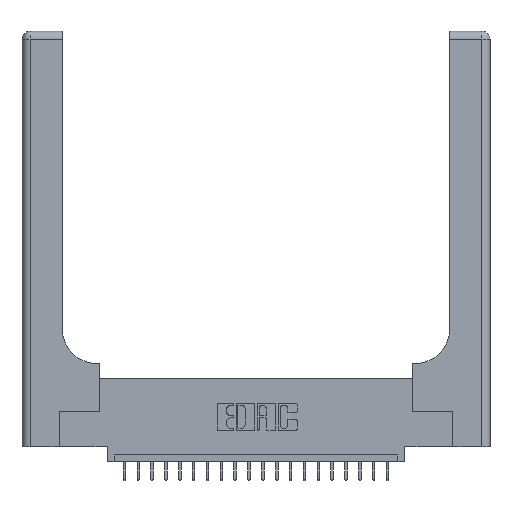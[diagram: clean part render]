
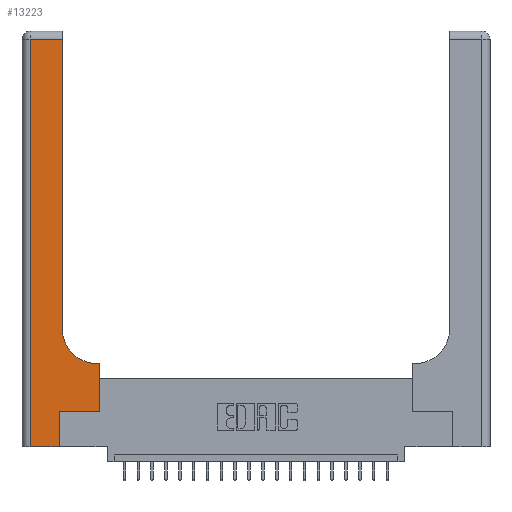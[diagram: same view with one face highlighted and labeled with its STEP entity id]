
A CAD part, top view. The second image highlights one B-rep face of the part: STEP entity #13223.
In plain terms, the highlighted planar face has unit normal (0, 0, 1).
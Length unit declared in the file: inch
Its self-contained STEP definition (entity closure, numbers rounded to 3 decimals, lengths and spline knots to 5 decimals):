
#130 = ORIENTED_EDGE ( 'NONE', *, *, #7487, .T. ) ;
#332 = CARTESIAN_POINT ( 'NONE',  ( 0.06, 0., 0.37 ) ) ;
#352 = AXIS2_PLACEMENT_3D ( 'NONE', #9188, #16458, #19156 ) ;
#564 = EDGE_CURVE ( 'NONE', #5405, #22552, #14140, .T. ) ;
#884 = CARTESIAN_POINT ( 'NONE',  ( 0.5585, 0.6, 0.37 ) ) ;
#927 = DIRECTION ( 'NONE',  ( -1., 0., 0. ) ) ;
#1056 = CARTESIAN_POINT ( 'NONE',  ( 0.2915, 0.6, 0.37 ) ) ;
#1364 = CARTESIAN_POINT ( 'NONE',  ( 0.5585, 0.25, 0.37 ) ) ;
#1836 = PLANE ( 'NONE',  #352 ) ;
#2170 = VERTEX_POINT ( 'NONE', #17887 ) ;
#2450 = LINE ( 'NONE', #22140, #11781 ) ;
#2534 = EDGE_CURVE ( 'NONE', #4818, #21847, #2450, .T. ) ;
#3393 = VERTEX_POINT ( 'NONE', #13955 ) ;
#4415 = LINE ( 'NONE', #22246, #14226 ) ;
#4580 = VERTEX_POINT ( 'NONE', #332 ) ;
#4818 = VERTEX_POINT ( 'NONE', #6600 ) ;
#5195 = VECTOR ( 'NONE', #21370, 39.37008 ) ;
#5405 = VERTEX_POINT ( 'NONE', #1364 ) ;
#5787 = ORIENTED_EDGE ( 'NONE', *, *, #16520, .T. ) ;
#5951 = FACE_OUTER_BOUND ( 'NONE', #8430, .T. ) ;
#6069 = EDGE_CURVE ( 'NONE', #15256, #13187, #13491, .T. ) ;
#6600 = CARTESIAN_POINT ( 'NONE',  ( 0.269, 0., 0.37 ) ) ;
#7013 = DIRECTION ( 'NONE',  ( 0., 1., 0. ) ) ;
#7487 = EDGE_CURVE ( 'NONE', #21847, #5405, #16011, .T. ) ;
#7909 = CARTESIAN_POINT ( 'NONE',  ( 0., 2.94, 0.37 ) ) ;
#8078 = VECTOR ( 'NONE', #12597, 39.37008 ) ;
#8288 = VECTOR ( 'NONE', #21776, 39.37008 ) ;
#8430 = EDGE_LOOP ( 'NONE', ( #8604, #16390, #15786, #5787, #19103, #130, #19903, #15740, #17509 ) ) ;
#8604 = ORIENTED_EDGE ( 'NONE', *, *, #13156, .T. ) ;
#8641 = EDGE_CURVE ( 'NONE', #22552, #2170, #11867, .T. ) ;
#9188 = CARTESIAN_POINT ( 'NONE',  ( 0., 3., 0.37 ) ) ;
#9488 = EDGE_CURVE ( 'NONE', #13187, #4580, #4415, .T. ) ;
#10197 = DIRECTION ( 'NONE',  ( -1., 0., 0. ) ) ;
#10296 = CARTESIAN_POINT ( 'NONE',  ( 0.2915, 2.94, 0.37 ) ) ;
#10298 = VECTOR ( 'NONE', #927, 39.37008 ) ;
#10690 = CARTESIAN_POINT ( 'NONE',  ( 0.5585, 0.25, 0.37 ) ) ;
#11186 = DIRECTION ( 'NONE',  ( 0., 0., -1. ) ) ;
#11340 = CARTESIAN_POINT ( 'NONE',  ( 0.06, 2.94, 0.37 ) ) ;
#11781 = VECTOR ( 'NONE', #7013, 39.37008 ) ;
#11867 = LINE ( 'NONE', #1056, #14597 ) ;
#12467 = CARTESIAN_POINT ( 'NONE',  ( 0., 0., 0.37 ) ) ;
#12597 = DIRECTION ( 'NONE',  ( 1., 0., 0. ) ) ;
#12977 = CARTESIAN_POINT ( 'NONE',  ( 0.2915, 3., 0.37 ) ) ;
#13156 = EDGE_CURVE ( 'NONE', #3393, #15256, #21890, .T. ) ;
#13187 = VERTEX_POINT ( 'NONE', #11340 ) ;
#13223 = ADVANCED_FACE ( 'NONE', ( #5951 ), #1836, .F. ) ;
#13491 = LINE ( 'NONE', #7909, #10298 ) ;
#13955 = CARTESIAN_POINT ( 'NONE',  ( 0.2915, 0.85, 0.37 ) ) ;
#14140 = LINE ( 'NONE', #10690, #5195 ) ;
#14226 = VECTOR ( 'NONE', #15375, 39.37008 ) ;
#14256 = DIRECTION ( 'NONE',  ( 1., 0., 0. ) ) ;
#14597 = VECTOR ( 'NONE', #10197, 39.37008 ) ;
#15256 = VERTEX_POINT ( 'NONE', #10296 ) ;
#15375 = DIRECTION ( 'NONE',  ( 0., -1., 0. ) ) ;
#15740 = ORIENTED_EDGE ( 'NONE', *, *, #8641, .T. ) ;
#15786 = ORIENTED_EDGE ( 'NONE', *, *, #9488, .T. ) ;
#16011 = LINE ( 'NONE', #23325, #17969 ) ;
#16390 = ORIENTED_EDGE ( 'NONE', *, *, #6069, .T. ) ;
#16458 = DIRECTION ( 'NONE',  ( 0., 0., -1. ) ) ;
#16520 = EDGE_CURVE ( 'NONE', #4580, #4818, #23374, .T. ) ;
#17509 = ORIENTED_EDGE ( 'NONE', *, *, #22043, .T. ) ;
#17887 = CARTESIAN_POINT ( 'NONE',  ( 0.5415, 0.6, 0.37 ) ) ;
#17969 = VECTOR ( 'NONE', #19240, 39.37008 ) ;
#18073 = CARTESIAN_POINT ( 'NONE',  ( 0.5415, 0.85, 0.37 ) ) ;
#19103 = ORIENTED_EDGE ( 'NONE', *, *, #2534, .T. ) ;
#19156 = DIRECTION ( 'NONE',  ( -1., 0., 0. ) ) ;
#19240 = DIRECTION ( 'NONE',  ( 1., 0., 0. ) ) ;
#19903 = ORIENTED_EDGE ( 'NONE', *, *, #564, .T. ) ;
#20127 = AXIS2_PLACEMENT_3D ( 'NONE', #18073, #11186, #14256 ) ;
#21370 = DIRECTION ( 'NONE',  ( 0., 1., 0. ) ) ;
#21776 = DIRECTION ( 'NONE',  ( 0., 1., 0. ) ) ;
#21847 = VERTEX_POINT ( 'NONE', #23244 ) ;
#21890 = LINE ( 'NONE', #12977, #8288 ) ;
#22043 = EDGE_CURVE ( 'NONE', #2170, #3393, #22371, .T. ) ;
#22140 = CARTESIAN_POINT ( 'NONE',  ( 0.269, 0., 0.37 ) ) ;
#22246 = CARTESIAN_POINT ( 'NONE',  ( 0.06, 3., 0.37 ) ) ;
#22371 = CIRCLE ( 'NONE', #20127, 0.25 ) ;
#22552 = VERTEX_POINT ( 'NONE', #884 ) ;
#23244 = CARTESIAN_POINT ( 'NONE',  ( 0.269, 0.25, 0.37 ) ) ;
#23325 = CARTESIAN_POINT ( 'NONE',  ( 0.269, 0.25, 0.37 ) ) ;
#23374 = LINE ( 'NONE', #12467, #8078 ) ;
